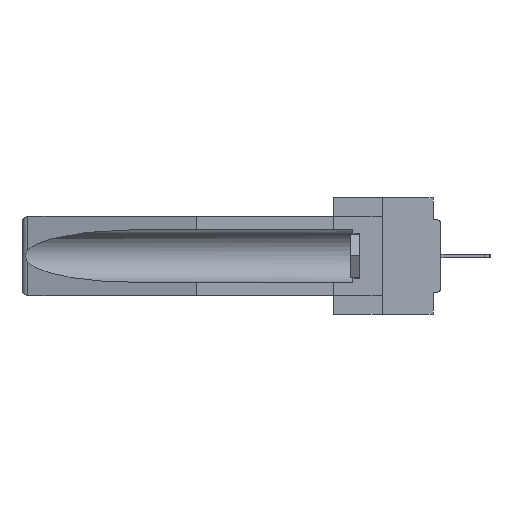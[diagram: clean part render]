
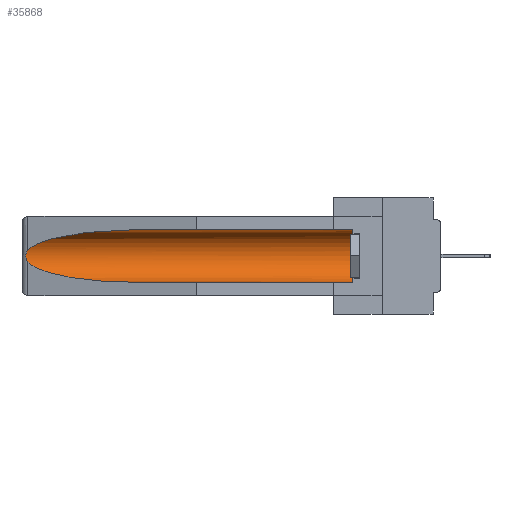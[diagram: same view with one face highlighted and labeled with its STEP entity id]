
A CAD part, left-side view. The second image highlights one B-rep face of the part: STEP entity #35868.
In plain terms, the highlighted cylindrical face has radius 2.857 mm (diameter 5.715 mm), a partial arc.
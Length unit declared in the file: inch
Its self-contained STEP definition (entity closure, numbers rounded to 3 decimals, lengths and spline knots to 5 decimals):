
#1146 = EDGE_CURVE ( 'NONE', #5634, #10330, #34370, .T. ) ;
#2507 = AXIS2_PLACEMENT_3D ( 'NONE', #25636, #37225, #22603 ) ;
#4601 = CARTESIAN_POINT ( 'NONE',  ( 0.25451, 1.48313, -0.24835 ) ) ;
#5447 = CARTESIAN_POINT ( 'NONE',  ( 0.26655, 1.53094, -0.18657 ) ) ;
#5483 = DIRECTION ( 'NONE',  ( 0., 1., 0. ) ) ;
#5634 = VERTEX_POINT ( 'NONE', #35296 ) ;
#5813 = EDGE_CURVE ( 'NONE', #5634, #16681, #22934, .T. ) ;
#6533 = AXIS2_PLACEMENT_3D ( 'NONE', #25212, #27682, #22555 ) ;
#7082 = CARTESIAN_POINT ( 'NONE',  ( 0.26537, 1.52718, -0.19328 ) ) ;
#7947 = CARTESIAN_POINT ( 'NONE',  ( 0.155, 1.07973, -0.059 ) ) ;
#8109 = CARTESIAN_POINT ( 'NONE',  ( 0.2673, 1.5327, -0.16383 ) ) ;
#8487 = ORIENTED_EDGE ( 'NONE', *, *, #29701, .T. ) ;
#9355 = EDGE_CURVE ( 'NONE', #16681, #22233, #23286, .T. ) ;
#9429 = CARTESIAN_POINT ( 'NONE',  ( 0.155, 1.07973, -0.059 ) ) ;
#10330 = VERTEX_POINT ( 'NONE', #35850 ) ;
#10605 =( BOUNDED_CURVE ( )  B_SPLINE_CURVE ( 3, ( #7082, #4601, #30262, #21338 ),
 .UNSPECIFIED., .F., .T. ) 
 B_SPLINE_CURVE_WITH_KNOTS ( ( 4, 4 ),
 ( 0.1948, 1.5708 ),
 .UNSPECIFIED. ) 
 CURVE ( )  GEOMETRIC_REPRESENTATION_ITEM ( )  RATIONAL_B_SPLINE_CURVE ( ( 1., 0.848, 0.848, 1. ) ) 
 REPRESENTATION_ITEM ( '' )  );
#10965 = ORIENTED_EDGE ( 'NONE', *, *, #32116, .T. ) ;
#12141 = CARTESIAN_POINT ( 'NONE',  ( 0.155, 0.126, -0.059 ) ) ;
#13275 = ORIENTED_EDGE ( 'NONE', *, *, #9355, .T. ) ;
#15485 = EDGE_LOOP ( 'NONE', ( #8487, #19864, #10965, #28857, #25698, #13275 ) ) ;
#16681 = VERTEX_POINT ( 'NONE', #12141 ) ;
#17123 = CARTESIAN_POINT ( 'NONE',  ( 0.25451, 1.48313, -0.09465 ) ) ;
#19736 = CYLINDRICAL_SURFACE ( 'NONE', #2507, 0.1125 ) ;
#19864 = ORIENTED_EDGE ( 'NONE', *, *, #27829, .T. ) ;
#20158 = VECTOR ( 'NONE', #5483, 39.37008 ) ;
#20945 = CARTESIAN_POINT ( 'NONE',  ( 0.2675, 1.53308, -0.16763 ) ) ;
#21036 = CARTESIAN_POINT ( 'NONE',  ( 0.26537, 1.52718, -0.14972 ) ) ;
#21338 = CARTESIAN_POINT ( 'NONE',  ( 0.155, 1.07973, -0.284 ) ) ;
#22233 = VERTEX_POINT ( 'NONE', #7947 ) ;
#22440 = B_SPLINE_CURVE_WITH_KNOTS ( 'NONE', 3,
 ( #31468, #28808, #23124, #8109, #20945, #31651, #34326, #5447, #25603, #37187 ),
 .UNSPECIFIED., .F., .F.,
 ( 4, 2, 2, 2, 4 ),
 ( 0., 0.00029, 0.00058, 0.00087, 0.00117 ),
 .UNSPECIFIED. ) ;
#22555 = DIRECTION ( 'NONE',  ( 0., 0., 1. ) ) ;
#22603 = DIRECTION ( 'NONE',  ( 0., 0., 1. ) ) ;
#22604 = CARTESIAN_POINT ( 'NONE',  ( 0.155, -0.30754, -0.284 ) ) ;
#22934 = CIRCLE ( 'NONE', #6533, 0.1125 ) ;
#22973 = FACE_OUTER_BOUND ( 'NONE', #15485, .T. ) ;
#23124 = CARTESIAN_POINT ( 'NONE',  ( 0.26654, 1.53092, -0.15636 ) ) ;
#23286 = LINE ( 'NONE', #29171, #32655 ) ;
#24277 = CARTESIAN_POINT ( 'NONE',  ( 0.21114, 1.30732, -0.059 ) ) ;
#24510 = CARTESIAN_POINT ( 'NONE',  ( 0.26537, 1.52718, -0.19328 ) ) ;
#25212 = CARTESIAN_POINT ( 'NONE',  ( 0.155, 0.126, -0.1715 ) ) ;
#25603 = CARTESIAN_POINT ( 'NONE',  ( 0.26597, 1.5296, -0.19026 ) ) ;
#25636 = CARTESIAN_POINT ( 'NONE',  ( 0.155, -0.30754, -0.1715 ) ) ;
#25698 = ORIENTED_EDGE ( 'NONE', *, *, #5813, .T. ) ;
#26592 = CARTESIAN_POINT ( 'NONE',  ( 0.26537, 1.52718, -0.14972 ) ) ;
#27097 = VERTEX_POINT ( 'NONE', #24510 ) ;
#27682 = DIRECTION ( 'NONE',  ( 0., -1., 0. ) ) ;
#27829 = EDGE_CURVE ( 'NONE', #33231, #27097, #22440, .T. ) ;
#28808 = CARTESIAN_POINT ( 'NONE',  ( 0.26597, 1.52961, -0.15275 ) ) ;
#28857 = ORIENTED_EDGE ( 'NONE', *, *, #1146, .F. ) ;
#28979 = DIRECTION ( 'NONE',  ( 0., 1., 0. ) ) ;
#29171 = CARTESIAN_POINT ( 'NONE',  ( 0.155, -0.30754, -0.059 ) ) ;
#29701 = EDGE_CURVE ( 'NONE', #22233, #33231, #32689, .T. ) ;
#30262 = CARTESIAN_POINT ( 'NONE',  ( 0.21114, 1.30732, -0.284 ) ) ;
#31468 = CARTESIAN_POINT ( 'NONE',  ( 0.26537, 1.52718, -0.14972 ) ) ;
#31651 = CARTESIAN_POINT ( 'NONE',  ( 0.2675, 1.53308, -0.17534 ) ) ;
#32116 = EDGE_CURVE ( 'NONE', #27097, #10330, #10605, .T. ) ;
#32655 = VECTOR ( 'NONE', #28979, 39.37008 ) ;
#32689 =( BOUNDED_CURVE ( )  B_SPLINE_CURVE ( 3, ( #9429, #24277, #17123, #21036 ),
 .UNSPECIFIED., .F., .T. ) 
 B_SPLINE_CURVE_WITH_KNOTS ( ( 4, 4 ),
 ( 4.71239, 6.08839 ),
 .UNSPECIFIED. ) 
 CURVE ( )  GEOMETRIC_REPRESENTATION_ITEM ( )  RATIONAL_B_SPLINE_CURVE ( ( 1., 0.848, 0.848, 1. ) ) 
 REPRESENTATION_ITEM ( '' )  );
#33231 = VERTEX_POINT ( 'NONE', #26592 ) ;
#34326 = CARTESIAN_POINT ( 'NONE',  ( 0.2673, 1.53269, -0.17917 ) ) ;
#34370 = LINE ( 'NONE', #22604, #20158 ) ;
#35296 = CARTESIAN_POINT ( 'NONE',  ( 0.155, 0.126, -0.284 ) ) ;
#35850 = CARTESIAN_POINT ( 'NONE',  ( 0.155, 1.07973, -0.284 ) ) ;
#35868 = ADVANCED_FACE ( 'NONE', ( #22973 ), #19736, .F. ) ;
#37187 = CARTESIAN_POINT ( 'NONE',  ( 0.26537, 1.52718, -0.19328 ) ) ;
#37225 = DIRECTION ( 'NONE',  ( 0., 1., 0. ) ) ;
